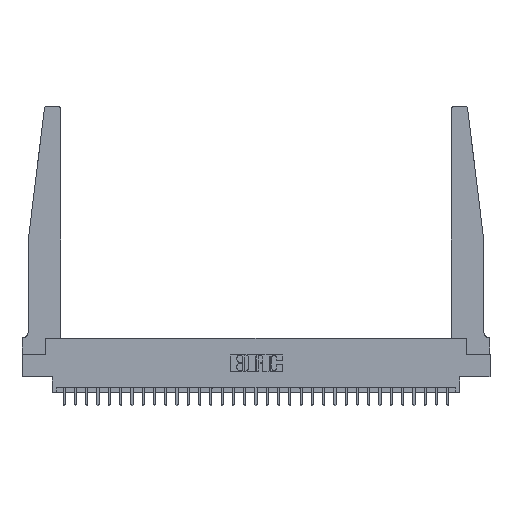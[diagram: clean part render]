
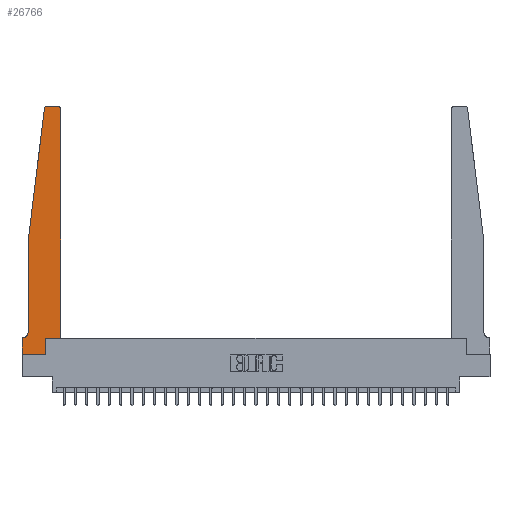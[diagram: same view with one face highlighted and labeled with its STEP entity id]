
A CAD part, top view. The second image highlights one B-rep face of the part: STEP entity #26766.
In plain terms, the highlighted planar face has unit normal (0, 0, 1).
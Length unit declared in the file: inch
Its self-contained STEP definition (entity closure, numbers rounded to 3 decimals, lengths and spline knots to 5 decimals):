
#54 = DIRECTION ( 'NONE',  ( 1., 0., 0. ) ) ;
#123 = CARTESIAN_POINT ( 'NONE',  ( 0.27653, 2.72, 0.37 ) ) ;
#220 = CARTESIAN_POINT ( 'NONE',  ( 0.065, 0.1875, 0.37 ) ) ;
#501 = AXIS2_PLACEMENT_3D ( 'NONE', #123, #15783, #2376 ) ;
#644 = CARTESIAN_POINT ( 'NONE',  ( 0., 0., 0.37 ) ) ;
#1002 = EDGE_CURVE ( 'NONE', #12980, #1383, #20865, .T. ) ;
#1325 = CARTESIAN_POINT ( 'NONE',  ( 0.25, 2.75, 0.37 ) ) ;
#1383 = VERTEX_POINT ( 'NONE', #3018 ) ;
#1698 = FACE_OUTER_BOUND ( 'NONE', #28400, .T. ) ;
#1731 = DIRECTION ( 'NONE',  ( 0., 0., -1. ) ) ;
#2376 = DIRECTION ( 'NONE',  ( 1., 0., 0. ) ) ;
#2409 = PLANE ( 'NONE',  #12208 ) ;
#2826 = ORIENTED_EDGE ( 'NONE', *, *, #1002, .T. ) ;
#2865 = VERTEX_POINT ( 'NONE', #16673 ) ;
#2871 = CARTESIAN_POINT ( 'NONE',  ( 0., 0., 0.37 ) ) ;
#3018 = CARTESIAN_POINT ( 'NONE',  ( 0.395, 2.75, 0.37 ) ) ;
#3901 = VECTOR ( 'NONE', #16241, 39.37008 ) ;
#3909 = VECTOR ( 'NONE', #4077, 39.37008 ) ;
#4009 = VERTEX_POINT ( 'NONE', #13974 ) ;
#4077 = DIRECTION ( 'NONE',  ( -0.122, -0.992, 0. ) ) ;
#4423 = ORIENTED_EDGE ( 'NONE', *, *, #19427, .T. ) ;
#4781 = DIRECTION ( 'NONE',  ( 1., 0., 0. ) ) ;
#5178 = VECTOR ( 'NONE', #20799, 39.37008 ) ;
#5463 = EDGE_CURVE ( 'NONE', #11100, #20000, #26610, .T. ) ;
#5616 = CARTESIAN_POINT ( 'NONE',  ( 0.27653, 2.75, 0.37 ) ) ;
#6218 = EDGE_CURVE ( 'NONE', #18164, #12980, #9307, .T. ) ;
#6361 = VECTOR ( 'NONE', #16884, 39.37008 ) ;
#6456 = ORIENTED_EDGE ( 'NONE', *, *, #27358, .T. ) ;
#7362 = AXIS2_PLACEMENT_3D ( 'NONE', #26710, #13510, #54 ) ;
#7393 = ORIENTED_EDGE ( 'NONE', *, *, #12251, .T. ) ;
#7766 = ORIENTED_EDGE ( 'NONE', *, *, #26502, .T. ) ;
#8094 = DIRECTION ( 'NONE',  ( 0., -1., 0. ) ) ;
#8199 = DIRECTION ( 'NONE',  ( -1., 0., 0. ) ) ;
#8216 = VERTEX_POINT ( 'NONE', #28703 ) ;
#9014 = VECTOR ( 'NONE', #9229, 39.37008 ) ;
#9229 = DIRECTION ( 'NONE',  ( -1., 0., 0. ) ) ;
#9238 = CARTESIAN_POINT ( 'NONE',  ( 0.425, 2.72, 0.37 ) ) ;
#9307 = LINE ( 'NONE', #26923, #20444 ) ;
#10076 = CARTESIAN_POINT ( 'NONE',  ( 0., 0.1875, 0.37 ) ) ;
#10089 = CARTESIAN_POINT ( 'NONE',  ( 0.2605, 0.18, 0.37 ) ) ;
#10929 = CARTESIAN_POINT ( 'NONE',  ( 0.065, 1.25, 0.37 ) ) ;
#11100 = VERTEX_POINT ( 'NONE', #15310 ) ;
#11198 = LINE ( 'NONE', #2871, #5178 ) ;
#11814 = ORIENTED_EDGE ( 'NONE', *, *, #13783, .T. ) ;
#12073 = CARTESIAN_POINT ( 'NONE',  ( 0.065, 0.2375, 0.37 ) ) ;
#12208 = AXIS2_PLACEMENT_3D ( 'NONE', #15929, #18201, #4781 ) ;
#12251 = EDGE_CURVE ( 'NONE', #15296, #11100, #26477, .T. ) ;
#12615 = VECTOR ( 'NONE', #24588, 39.37008 ) ;
#12980 = VERTEX_POINT ( 'NONE', #9238 ) ;
#13286 = LINE ( 'NONE', #17964, #12615 ) ;
#13316 = VECTOR ( 'NONE', #8199, 39.37008 ) ;
#13510 = DIRECTION ( 'NONE',  ( 0., 0., 1. ) ) ;
#13783 = EDGE_CURVE ( 'NONE', #16032, #18164, #13286, .T. ) ;
#13974 = CARTESIAN_POINT ( 'NONE',  ( 0.24675, 2.72367, 0.37 ) ) ;
#13995 = LINE ( 'NONE', #1325, #13316 ) ;
#14201 = VERTEX_POINT ( 'NONE', #22007 ) ;
#14945 = ORIENTED_EDGE ( 'NONE', *, *, #20198, .T. ) ;
#15160 = CARTESIAN_POINT ( 'NONE',  ( 0.015, 0.2375, 0.37 ) ) ;
#15296 = VERTEX_POINT ( 'NONE', #12073 ) ;
#15310 = CARTESIAN_POINT ( 'NONE',  ( 0.015, 0.1875, 0.37 ) ) ;
#15318 = CIRCLE ( 'NONE', #501, 0.03 ) ;
#15783 = DIRECTION ( 'NONE',  ( 0., 0., 1. ) ) ;
#15802 = LINE ( 'NONE', #644, #3901 ) ;
#15929 = CARTESIAN_POINT ( 'NONE',  ( 0., 0.1875, 0.37 ) ) ;
#16032 = VERTEX_POINT ( 'NONE', #10089 ) ;
#16236 = ORIENTED_EDGE ( 'NONE', *, *, #25253, .T. ) ;
#16241 = DIRECTION ( 'NONE',  ( 0., -1., 0. ) ) ;
#16351 = ORIENTED_EDGE ( 'NONE', *, *, #26540, .T. ) ;
#16673 = CARTESIAN_POINT ( 'NONE',  ( 0., 0., 0.37 ) ) ;
#16882 = VERTEX_POINT ( 'NONE', #5616 ) ;
#16884 = DIRECTION ( 'NONE',  ( 0., 1., 0. ) ) ;
#17435 = DIRECTION ( 'NONE',  ( -1., 0., 0. ) ) ;
#17964 = CARTESIAN_POINT ( 'NONE',  ( 0.425, 0.18, 0.37 ) ) ;
#18164 = VERTEX_POINT ( 'NONE', #27427 ) ;
#18201 = DIRECTION ( 'NONE',  ( 0., 0., 1. ) ) ;
#18222 = DIRECTION ( 'NONE',  ( 0., 1., 0. ) ) ;
#19427 = EDGE_CURVE ( 'NONE', #20000, #2865, #15802, .T. ) ;
#20000 = VERTEX_POINT ( 'NONE', #10076 ) ;
#20198 = EDGE_CURVE ( 'NONE', #4009, #8216, #21770, .T. ) ;
#20444 = VECTOR ( 'NONE', #18222, 39.37008 ) ;
#20799 = DIRECTION ( 'NONE',  ( 1., 0., 0. ) ) ;
#20865 = CIRCLE ( 'NONE', #7362, 0.03 ) ;
#21770 = LINE ( 'NONE', #10929, #3909 ) ;
#22007 = CARTESIAN_POINT ( 'NONE',  ( 0.2605, 0., 0.37 ) ) ;
#22012 = ORIENTED_EDGE ( 'NONE', *, *, #6218, .T. ) ;
#23563 = CARTESIAN_POINT ( 'NONE',  ( 0.2605, 0.18, 0.37 ) ) ;
#24084 = LINE ( 'NONE', #23563, #6361 ) ;
#24546 = AXIS2_PLACEMENT_3D ( 'NONE', #15160, #1731, #17435 ) ;
#24588 = DIRECTION ( 'NONE',  ( 1., 0., 0. ) ) ;
#25252 = ORIENTED_EDGE ( 'NONE', *, *, #27516, .T. ) ;
#25253 = EDGE_CURVE ( 'NONE', #14201, #16032, #24084, .T. ) ;
#25761 = LINE ( 'NONE', #25783, #26425 ) ;
#25783 = CARTESIAN_POINT ( 'NONE',  ( 0.065, 1.25, 0.37 ) ) ;
#26425 = VECTOR ( 'NONE', #8094, 39.37008 ) ;
#26477 = CIRCLE ( 'NONE', #24546, 0.05 ) ;
#26502 = EDGE_CURVE ( 'NONE', #8216, #15296, #25761, .T. ) ;
#26540 = EDGE_CURVE ( 'NONE', #1383, #16882, #13995, .T. ) ;
#26610 = LINE ( 'NONE', #220, #9014 ) ;
#26710 = CARTESIAN_POINT ( 'NONE',  ( 0.395, 2.72, 0.37 ) ) ;
#26766 = ADVANCED_FACE ( 'NONE', ( #1698 ), #2409, .T. ) ;
#26923 = CARTESIAN_POINT ( 'NONE',  ( 0.425, 0.18, 0.37 ) ) ;
#27358 = EDGE_CURVE ( 'NONE', #16882, #4009, #15318, .T. ) ;
#27427 = CARTESIAN_POINT ( 'NONE',  ( 0.425, 0.18, 0.37 ) ) ;
#27516 = EDGE_CURVE ( 'NONE', #2865, #14201, #11198, .T. ) ;
#28400 = EDGE_LOOP ( 'NONE', ( #16351, #6456, #14945, #7766, #7393, #28612, #4423, #25252, #16236, #11814, #22012, #2826 ) ) ;
#28612 = ORIENTED_EDGE ( 'NONE', *, *, #5463, .T. ) ;
#28703 = CARTESIAN_POINT ( 'NONE',  ( 0.065, 1.25, 0.37 ) ) ;
